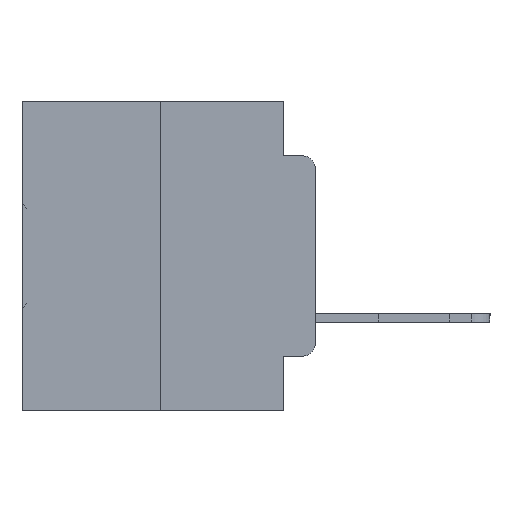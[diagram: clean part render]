
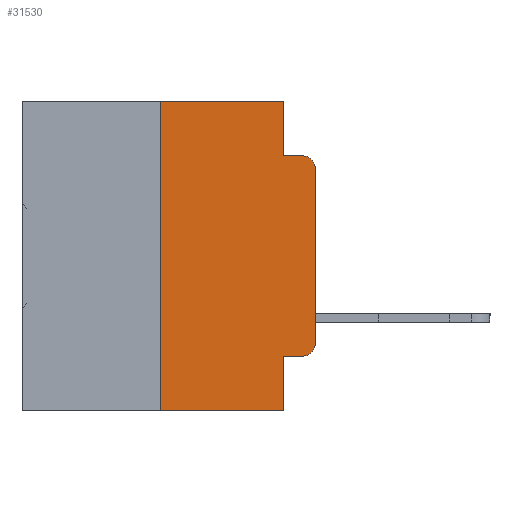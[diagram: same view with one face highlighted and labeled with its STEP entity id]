
A CAD part, left-side view. The second image highlights one B-rep face of the part: STEP entity #31530.
In plain terms, the highlighted planar face has unit normal (-1, 0, 0).
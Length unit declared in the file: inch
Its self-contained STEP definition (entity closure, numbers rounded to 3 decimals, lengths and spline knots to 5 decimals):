
#320 = CARTESIAN_POINT ( 'NONE',  ( 0., 0., -0.1085 ) ) ;
#360 = EDGE_CURVE ( 'NONE', #4331, #11701, #15287, .T. ) ;
#754 = LINE ( 'NONE', #30213, #4354 ) ;
#1316 = CARTESIAN_POINT ( 'NONE',  ( 0., 0.473, 0. ) ) ;
#2470 = DIRECTION ( 'NONE',  ( 0., -1., 0. ) ) ;
#2732 = DIRECTION ( 'NONE',  ( 0., 0., 1. ) ) ;
#2949 = CARTESIAN_POINT ( 'NONE',  ( 0., 0.051, -0.0885 ) ) ;
#3804 = EDGE_CURVE ( 'NONE', #4331, #32418, #23794, .T. ) ;
#3904 = LINE ( 'NONE', #1316, #24106 ) ;
#4331 = VERTEX_POINT ( 'NONE', #7517 ) ;
#4354 = VECTOR ( 'NONE', #2470, 39.37008 ) ;
#4685 = ORIENTED_EDGE ( 'NONE', *, *, #18453, .T. ) ;
#4901 = CARTESIAN_POINT ( 'NONE',  ( 0., 0.051, -0.4115 ) ) ;
#5354 = CARTESIAN_POINT ( 'NONE',  ( 0., 0.051, 0. ) ) ;
#5782 = CARTESIAN_POINT ( 'NONE',  ( 0., 0.02, -0.0885 ) ) ;
#6174 = DIRECTION ( 'NONE',  ( 0., 0., -1. ) ) ;
#6201 = ORIENTED_EDGE ( 'NONE', *, *, #23678, .T. ) ;
#6359 = AXIS2_PLACEMENT_3D ( 'NONE', #11844, #29462, #14356 ) ;
#6435 = DIRECTION ( 'NONE',  ( 0., -1., 0. ) ) ;
#7136 = CARTESIAN_POINT ( 'NONE',  ( 0., 0.02, -0.4115 ) ) ;
#7517 = CARTESIAN_POINT ( 'NONE',  ( 0., 0.051, -0.4115 ) ) ;
#8127 = VERTEX_POINT ( 'NONE', #5782 ) ;
#8543 = LINE ( 'NONE', #18814, #14520 ) ;
#8623 = DIRECTION ( 'NONE',  ( 0., -1., 0. ) ) ;
#9061 = CIRCLE ( 'NONE', #6359, 0.02 ) ;
#9397 = CARTESIAN_POINT ( 'NONE',  ( 0., 0.25, -0.5 ) ) ;
#10365 = VECTOR ( 'NONE', #8623, 39.37008 ) ;
#10538 = DIRECTION ( 'NONE',  ( 0., 0., 1. ) ) ;
#10883 = PLANE ( 'NONE',  #22044 ) ;
#11422 = CIRCLE ( 'NONE', #12753, 0.02 ) ;
#11454 = VERTEX_POINT ( 'NONE', #320 ) ;
#11701 = VERTEX_POINT ( 'NONE', #31905 ) ;
#11844 = CARTESIAN_POINT ( 'NONE',  ( 0., 0.02, -0.1085 ) ) ;
#12353 = LINE ( 'NONE', #12979, #19826 ) ;
#12627 = VERTEX_POINT ( 'NONE', #2949 ) ;
#12753 = AXIS2_PLACEMENT_3D ( 'NONE', #15139, #32688, #17690 ) ;
#12979 = CARTESIAN_POINT ( 'NONE',  ( 0., 0.473, -0.5 ) ) ;
#13355 = EDGE_LOOP ( 'NONE', ( #24025, #6201, #27975, #20867, #24473, #14191, #4685, #24500, #28448, #19775 ) ) ;
#13411 = DIRECTION ( 'NONE',  ( 1., 0., 0. ) ) ;
#14191 = ORIENTED_EDGE ( 'NONE', *, *, #29846, .F. ) ;
#14356 = DIRECTION ( 'NONE',  ( 0., 0., -1. ) ) ;
#14520 = VECTOR ( 'NONE', #6174, 39.37008 ) ;
#15139 = CARTESIAN_POINT ( 'NONE',  ( 0., 0.02, -0.3915 ) ) ;
#15287 = LINE ( 'NONE', #5354, #21217 ) ;
#16556 = VERTEX_POINT ( 'NONE', #25713 ) ;
#16804 = DIRECTION ( 'NONE',  ( 0., 0., -1. ) ) ;
#17491 = CARTESIAN_POINT ( 'NONE',  ( 0., 0.051, 0. ) ) ;
#17690 = DIRECTION ( 'NONE',  ( 0., 0., -1. ) ) ;
#17859 = LINE ( 'NONE', #17935, #25358 ) ;
#17935 = CARTESIAN_POINT ( 'NONE',  ( 0., 0., 0. ) ) ;
#18453 = EDGE_CURVE ( 'NONE', #26527, #11701, #12353, .T. ) ;
#18814 = CARTESIAN_POINT ( 'NONE',  ( 0., 0.051, 0. ) ) ;
#19331 = EDGE_CURVE ( 'NONE', #16556, #29701, #3904, .T. ) ;
#19775 = ORIENTED_EDGE ( 'NONE', *, *, #20148, .T. ) ;
#19826 = VECTOR ( 'NONE', #22995, 39.37008 ) ;
#20070 = CARTESIAN_POINT ( 'NONE',  ( 0., 0., -0.3915 ) ) ;
#20148 = EDGE_CURVE ( 'NONE', #32418, #20753, #11422, .T. ) ;
#20753 = VERTEX_POINT ( 'NONE', #20070 ) ;
#20867 = ORIENTED_EDGE ( 'NONE', *, *, #24798, .F. ) ;
#21217 = VECTOR ( 'NONE', #16804, 39.37008 ) ;
#22044 = AXIS2_PLACEMENT_3D ( 'NONE', #26003, #13411, #30993 ) ;
#22995 = DIRECTION ( 'NONE',  ( 0., -1., 0. ) ) ;
#23678 = EDGE_CURVE ( 'NONE', #11454, #8127, #9061, .T. ) ;
#23794 = LINE ( 'NONE', #4901, #10365 ) ;
#24025 = ORIENTED_EDGE ( 'NONE', *, *, #28021, .T. ) ;
#24106 = VECTOR ( 'NONE', #6435, 39.37008 ) ;
#24473 = ORIENTED_EDGE ( 'NONE', *, *, #19331, .F. ) ;
#24500 = ORIENTED_EDGE ( 'NONE', *, *, #360, .F. ) ;
#24798 = EDGE_CURVE ( 'NONE', #29701, #12627, #8543, .T. ) ;
#25235 = LINE ( 'NONE', #25655, #26841 ) ;
#25358 = VECTOR ( 'NONE', #2732, 39.37008 ) ;
#25655 = CARTESIAN_POINT ( 'NONE',  ( 0., 0.25, 0. ) ) ;
#25713 = CARTESIAN_POINT ( 'NONE',  ( 0., 0.25, 0. ) ) ;
#26003 = CARTESIAN_POINT ( 'NONE',  ( 0., 0.473, 0. ) ) ;
#26527 = VERTEX_POINT ( 'NONE', #9397 ) ;
#26841 = VECTOR ( 'NONE', #10538, 39.37008 ) ;
#27975 = ORIENTED_EDGE ( 'NONE', *, *, #28485, .F. ) ;
#28021 = EDGE_CURVE ( 'NONE', #20753, #11454, #17859, .T. ) ;
#28448 = ORIENTED_EDGE ( 'NONE', *, *, #3804, .T. ) ;
#28485 = EDGE_CURVE ( 'NONE', #12627, #8127, #754, .T. ) ;
#29462 = DIRECTION ( 'NONE',  ( -1., 0., 0. ) ) ;
#29701 = VERTEX_POINT ( 'NONE', #17491 ) ;
#29846 = EDGE_CURVE ( 'NONE', #26527, #16556, #25235, .T. ) ;
#30213 = CARTESIAN_POINT ( 'NONE',  ( 0., 0.051, -0.0885 ) ) ;
#30971 = FACE_OUTER_BOUND ( 'NONE', #13355, .T. ) ;
#30993 = DIRECTION ( 'NONE',  ( 0., 0., -1. ) ) ;
#31530 = ADVANCED_FACE ( 'NONE', ( #30971 ), #10883, .F. ) ;
#31905 = CARTESIAN_POINT ( 'NONE',  ( 0., 0.051, -0.5 ) ) ;
#32418 = VERTEX_POINT ( 'NONE', #7136 ) ;
#32688 = DIRECTION ( 'NONE',  ( -1., 0., 0. ) ) ;
